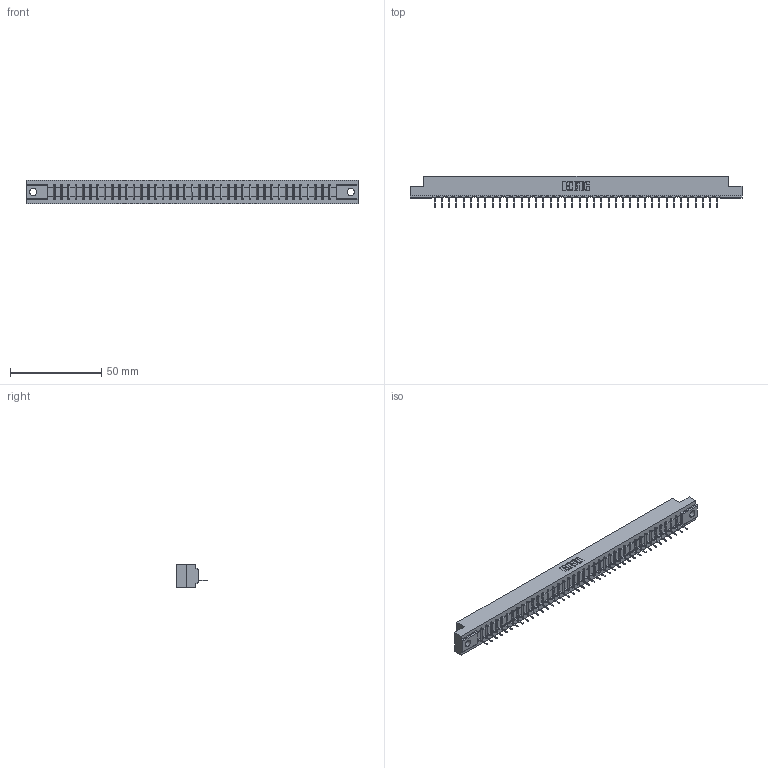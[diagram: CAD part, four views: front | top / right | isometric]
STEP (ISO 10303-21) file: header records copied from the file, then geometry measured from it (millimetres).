
FILE_DESCRIPTION (( 'STEP AP203' ), '1' );
FILE_NAME ('307-040-431-104.STEP', '2020-09-29T09:31:03', ( '' ), ( '' ), 'SwSTEP 2.0', 'SolidWorks 2020', '' );
FILE_SCHEMA (( 'CONFIG_CONTROL_DESIGN' ));
Length unit declared in the file: inch
Products named in the file (3): 307-040-431-104; 307 Part_.156 Dia Mounting Holes; 307-290-001_531
Assembly tree (41 placements, depth 2):
  307-040-431-104
    307 Part_.156 Dia Mounting Holes
    307-290-001_531  x40
Bounding box: 181.51 x 17.42 x 12.7 mm (x, y, z)
Volume: 18652.1 mm3; surface area: 19090.4 mm2
Topology: 41 solids, 41 shells, 2413 faces, 6839 edges, 4394 vertices
Faces by surface type: plane 1564, cylinder 767, sphere 82
Entity records: 34924 total; most frequent: CARTESIAN_POINT 5886, ORIENTED_EDGE 5870, DIRECTION 5717, EDGE_CURVE 2935, VECTOR 2259, LINE 2259, VERTEX_POINT 1898, AXIS2_PLACEMENT_3D 1729
